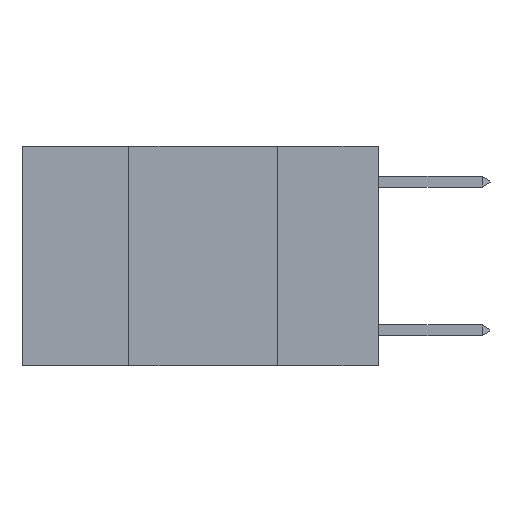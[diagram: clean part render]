
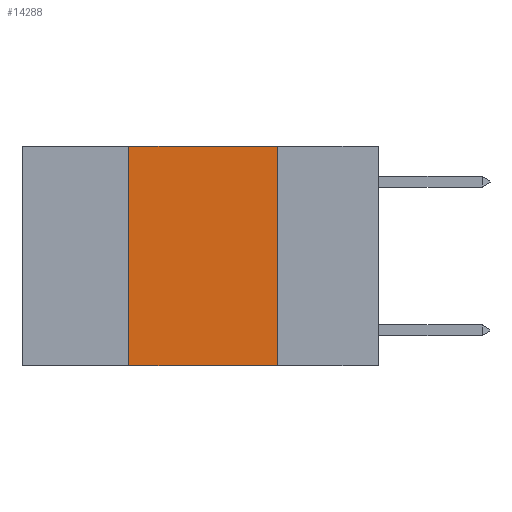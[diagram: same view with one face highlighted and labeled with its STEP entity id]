
A CAD part, left-side view. The second image highlights one B-rep face of the part: STEP entity #14288.
In plain terms, the highlighted planar face has unit normal (-1, 0, 0).
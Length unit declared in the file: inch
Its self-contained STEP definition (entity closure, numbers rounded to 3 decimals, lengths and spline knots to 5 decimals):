
#224 = LINE ( 'NONE', #5864, #5883 ) ;
#408 = EDGE_LOOP ( 'NONE', ( #9343, #23654, #27112, #5625 ) ) ;
#2590 = AXIS2_PLACEMENT_3D ( 'NONE', #12717, #29620, #15128 ) ;
#2615 = LINE ( 'NONE', #11745, #14687 ) ;
#3012 = CARTESIAN_POINT ( 'NONE',  ( 0., 0.42, -0.37 ) ) ;
#5625 = ORIENTED_EDGE ( 'NONE', *, *, #11819, .T. ) ;
#5864 = CARTESIAN_POINT ( 'NONE',  ( 0., 0.17, 0. ) ) ;
#5883 = VECTOR ( 'NONE', #8311, 39.37008 ) ;
#6890 = DIRECTION ( 'NONE',  ( 0., -1., 0. ) ) ;
#7416 = CARTESIAN_POINT ( 'NONE',  ( 0., 0.42, 0. ) ) ;
#8311 = DIRECTION ( 'NONE',  ( 0., 0., -1. ) ) ;
#8531 = VECTOR ( 'NONE', #17697, 39.37008 ) ;
#9030 = FACE_OUTER_BOUND ( 'NONE', #408, .T. ) ;
#9343 = ORIENTED_EDGE ( 'NONE', *, *, #15787, .F. ) ;
#11745 = CARTESIAN_POINT ( 'NONE',  ( 0., 0.42, 0. ) ) ;
#11819 = EDGE_CURVE ( 'NONE', #25665, #22569, #25397, .T. ) ;
#12717 = CARTESIAN_POINT ( 'NONE',  ( 0., 0.6, 0. ) ) ;
#12878 = CARTESIAN_POINT ( 'NONE',  ( 0., 0.6, 0. ) ) ;
#13836 = EDGE_CURVE ( 'NONE', #25665, #23167, #2615, .T. ) ;
#14288 = ADVANCED_FACE ( 'NONE', ( #9030 ), #27199, .F. ) ;
#14687 = VECTOR ( 'NONE', #26233, 39.37008 ) ;
#15128 = DIRECTION ( 'NONE',  ( 0., 0., -1. ) ) ;
#15689 = LINE ( 'NONE', #12878, #8531 ) ;
#15787 = EDGE_CURVE ( 'NONE', #18888, #22569, #224, .T. ) ;
#17697 = DIRECTION ( 'NONE',  ( 0., -1., 0. ) ) ;
#18888 = VERTEX_POINT ( 'NONE', #20396 ) ;
#18943 = VECTOR ( 'NONE', #6890, 39.37008 ) ;
#20396 = CARTESIAN_POINT ( 'NONE',  ( 0., 0.17, 0. ) ) ;
#22569 = VERTEX_POINT ( 'NONE', #27102 ) ;
#23167 = VERTEX_POINT ( 'NONE', #7416 ) ;
#23654 = ORIENTED_EDGE ( 'NONE', *, *, #29851, .F. ) ;
#25397 = LINE ( 'NONE', #28543, #18943 ) ;
#25665 = VERTEX_POINT ( 'NONE', #3012 ) ;
#26233 = DIRECTION ( 'NONE',  ( 0., 0., 1. ) ) ;
#27102 = CARTESIAN_POINT ( 'NONE',  ( 0., 0.17, -0.37 ) ) ;
#27112 = ORIENTED_EDGE ( 'NONE', *, *, #13836, .F. ) ;
#27199 = PLANE ( 'NONE',  #2590 ) ;
#28543 = CARTESIAN_POINT ( 'NONE',  ( 0., 0.6, -0.37 ) ) ;
#29620 = DIRECTION ( 'NONE',  ( 1., 0., 0. ) ) ;
#29851 = EDGE_CURVE ( 'NONE', #23167, #18888, #15689, .T. ) ;
